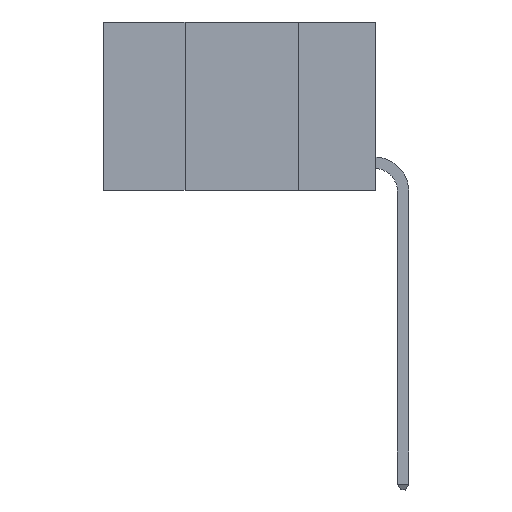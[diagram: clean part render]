
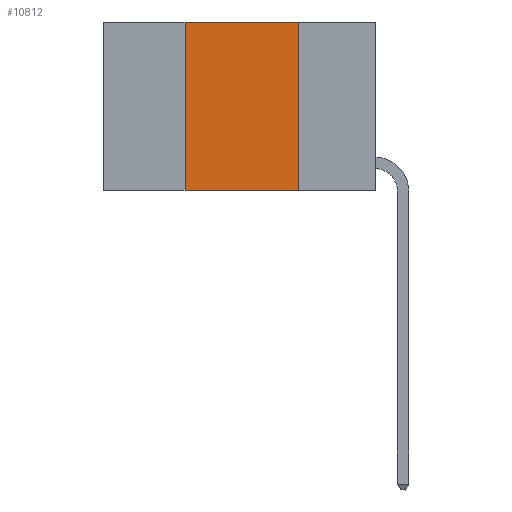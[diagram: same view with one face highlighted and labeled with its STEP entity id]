
A CAD part, left-side view. The second image highlights one B-rep face of the part: STEP entity #10812.
In plain terms, the highlighted planar face has unit normal (-1, 0, 0).
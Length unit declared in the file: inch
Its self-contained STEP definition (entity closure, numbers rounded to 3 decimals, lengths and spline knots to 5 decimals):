
#98 = CARTESIAN_POINT ( 'NONE',  ( 0., 0.6, -0.37 ) ) ;
#370 = VERTEX_POINT ( 'NONE', #15383 ) ;
#625 = AXIS2_PLACEMENT_3D ( 'NONE', #5900, #24096, #12104 ) ;
#1638 = EDGE_CURVE ( 'NONE', #370, #20183, #10885, .T. ) ;
#3536 = VECTOR ( 'NONE', #21819, 39.37008 ) ;
#3625 = LINE ( 'NONE', #98, #23867 ) ;
#4733 = DIRECTION ( 'NONE',  ( 0., -1., 0. ) ) ;
#5900 = CARTESIAN_POINT ( 'NONE',  ( 0., 0.6, 0. ) ) ;
#7895 = EDGE_CURVE ( 'NONE', #20183, #11304, #8961, .T. ) ;
#8773 = CARTESIAN_POINT ( 'NONE',  ( 0., 0.42, 0. ) ) ;
#8961 = LINE ( 'NONE', #9760, #3536 ) ;
#9442 = EDGE_CURVE ( 'NONE', #12832, #370, #19990, .T. ) ;
#9743 = CARTESIAN_POINT ( 'NONE',  ( 0., 0.17, 0. ) ) ;
#9760 = CARTESIAN_POINT ( 'NONE',  ( 0., 0.17, 0. ) ) ;
#10025 = PLANE ( 'NONE',  #625 ) ;
#10812 = ADVANCED_FACE ( 'NONE', ( #25854 ), #10025, .F. ) ;
#10846 = DIRECTION ( 'NONE',  ( 0., 0., 1. ) ) ;
#10885 = LINE ( 'NONE', #17140, #20948 ) ;
#11304 = VERTEX_POINT ( 'NONE', #15728 ) ;
#12104 = DIRECTION ( 'NONE',  ( 0., 0., -1. ) ) ;
#12473 = DIRECTION ( 'NONE',  ( 0., -1., 0. ) ) ;
#12832 = VERTEX_POINT ( 'NONE', #15812 ) ;
#13754 = EDGE_CURVE ( 'NONE', #12832, #11304, #3625, .T. ) ;
#14704 = VECTOR ( 'NONE', #10846, 39.37008 ) ;
#15383 = CARTESIAN_POINT ( 'NONE',  ( 0., 0.42, 0. ) ) ;
#15728 = CARTESIAN_POINT ( 'NONE',  ( 0., 0.17, -0.37 ) ) ;
#15812 = CARTESIAN_POINT ( 'NONE',  ( 0., 0.42, -0.37 ) ) ;
#15831 = ORIENTED_EDGE ( 'NONE', *, *, #9442, .F. ) ;
#17140 = CARTESIAN_POINT ( 'NONE',  ( 0., 0.6, 0. ) ) ;
#19575 = ORIENTED_EDGE ( 'NONE', *, *, #1638, .F. ) ;
#19990 = LINE ( 'NONE', #8773, #14704 ) ;
#20183 = VERTEX_POINT ( 'NONE', #9743 ) ;
#20948 = VECTOR ( 'NONE', #4733, 39.37008 ) ;
#21232 = EDGE_LOOP ( 'NONE', ( #21491, #19575, #15831, #24247 ) ) ;
#21491 = ORIENTED_EDGE ( 'NONE', *, *, #7895, .F. ) ;
#21819 = DIRECTION ( 'NONE',  ( 0., 0., -1. ) ) ;
#23867 = VECTOR ( 'NONE', #12473, 39.37008 ) ;
#24096 = DIRECTION ( 'NONE',  ( 1., 0., 0. ) ) ;
#24247 = ORIENTED_EDGE ( 'NONE', *, *, #13754, .T. ) ;
#25854 = FACE_OUTER_BOUND ( 'NONE', #21232, .T. ) ;
